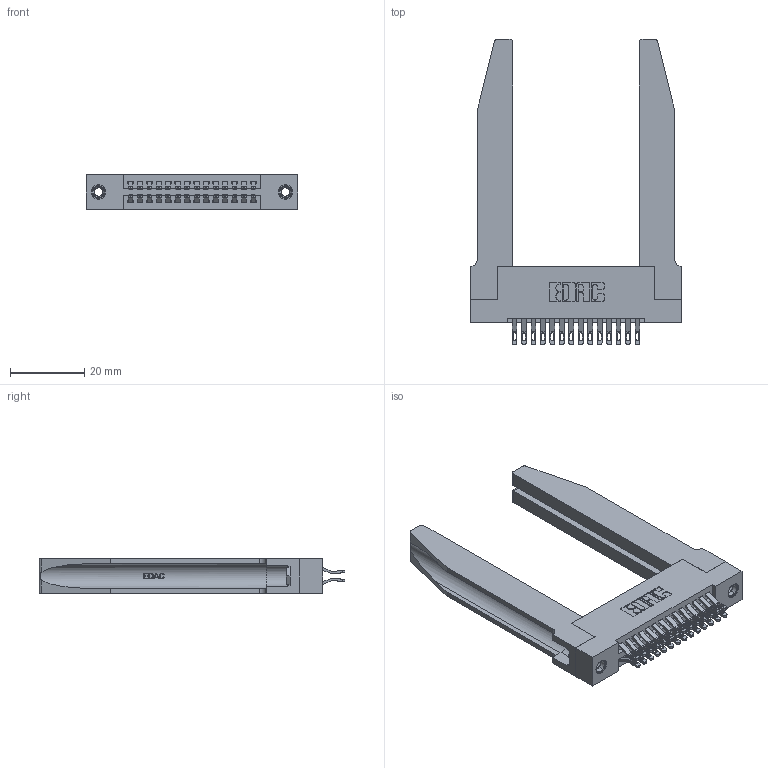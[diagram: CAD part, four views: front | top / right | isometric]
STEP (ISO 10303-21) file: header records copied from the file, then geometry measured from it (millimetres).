
FILE_DESCRIPTION (( 'STEP AP203' ), '1' );
FILE_NAME ('345-028-555-278.STEP', '2019-10-28T00:20:33', ( '' ), ( '' ), 'SwSTEP 2.0', 'SolidWorks 2016', '' );
FILE_SCHEMA (( 'CONFIG_CONTROL_DESIGN' ));
Length unit declared in the file: inch
Products named in the file (5): 345-028-555-278; 345-292-001_555 Tail; 345 Part_Flush Mounting Lugs - 0.156 Dia-TH; 345-250-001_345-250-001-102; 345-220-078_345-220-078
Assembly tree (33 placements, depth 2):
  345-028-555-278
    345 Part_Flush Mounting Lugs - 0.156 Dia-TH
    345-292-001_555 Tail  x28
    345-250-001_345-250-001-102  x2
    345-220-078_345-220-078  x2
Bounding box: 56.79 x 82.09 x 9.4 mm (x, y, z)
Volume: 13108.8 mm3; surface area: 14469.6 mm2
Topology: 33 solids, 33 shells, 1928 faces, 5905 edges, 3926 vertices
Faces by surface type: plane 1090, cylinder 786, bspline 36, cone 12, torus 4
Entity records: 19820 total; most frequent: CARTESIAN_POINT 4301, ORIENTED_EDGE 3102, DIRECTION 2789, EDGE_CURVE 1551, LINE 1249, VECTOR 1249, VERTEX_POINT 1028, AXIS2_PLACEMENT_3D 770
